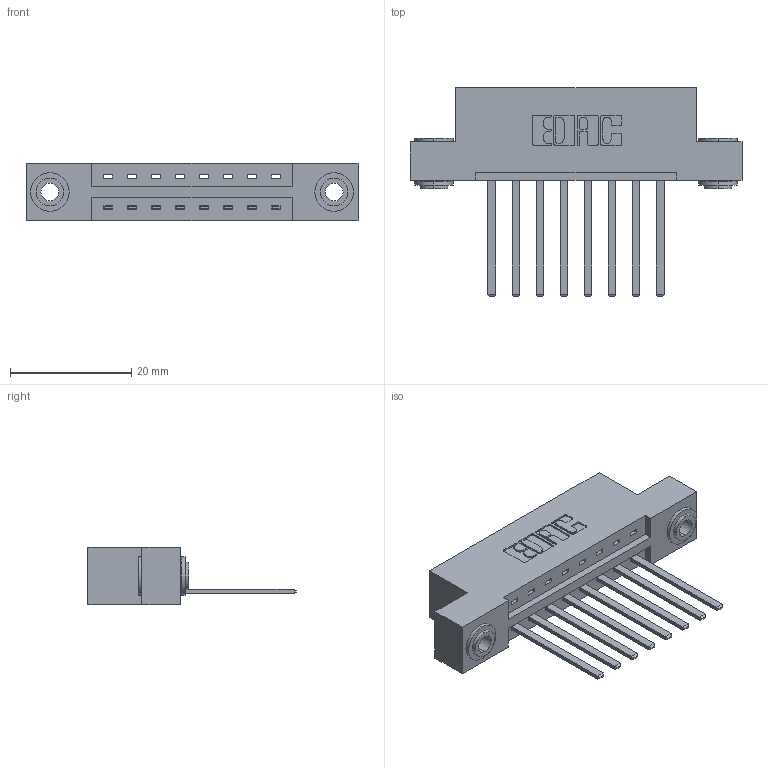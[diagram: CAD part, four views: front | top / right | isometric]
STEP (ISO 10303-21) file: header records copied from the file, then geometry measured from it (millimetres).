
FILE_DESCRIPTION (( 'STEP AP203' ), '1' );
FILE_NAME ('387-008-544-103.STEP', '2019-10-02T04:07:35', ( '' ), ( '' ), 'SwSTEP 2.0', 'SolidWorks 2016', '' );
FILE_SCHEMA (( 'CONFIG_CONTROL_DESIGN' ));
Length unit declared in the file: inch
Products named in the file (4): 387-008-544-103; 345-250-002_345-250-002-102; 345-292-001_345-293-144; 337 Part_Flush Mounting Lugs - 0.156 Dia-TH
Assembly tree (11 placements, depth 2):
  387-008-544-103
    337 Part_Flush Mounting Lugs - 0.156 Dia-TH
    345-292-001_345-293-144  x8
    345-250-002_345-250-002-102  x2
Bounding box: 54.71 x 34.3 x 9.4 mm (x, y, z)
Volume: 5372.9 mm3; surface area: 5900.9 mm2
Topology: 11 solids, 11 shells, 600 faces, 1747 edges, 1150 vertices
Faces by surface type: plane 416, cylinder 176, cone 8
Entity records: 10810 total; most frequent: CARTESIAN_POINT 1857, ORIENTED_EDGE 1794, DIRECTION 1663, EDGE_CURVE 897, VECTOR 749, LINE 749, VERTEX_POINT 594, AXIS2_PLACEMENT_3D 457
